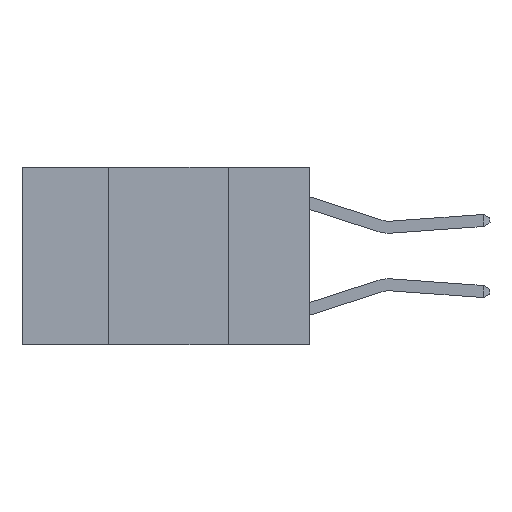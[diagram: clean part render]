
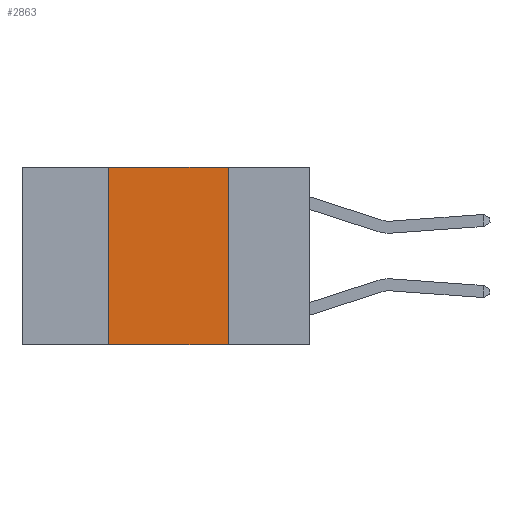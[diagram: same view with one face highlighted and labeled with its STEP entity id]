
A CAD part, left-side view. The second image highlights one B-rep face of the part: STEP entity #2863.
In plain terms, the highlighted planar face has unit normal (-1, 0, 0).
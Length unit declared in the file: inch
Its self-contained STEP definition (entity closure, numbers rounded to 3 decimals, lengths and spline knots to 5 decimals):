
#155 = VERTEX_POINT ( 'NONE', #14395 ) ;
#500 = DIRECTION ( 'NONE',  ( 0., -1., 0. ) ) ;
#673 = CARTESIAN_POINT ( 'NONE',  ( 0., 0.17, 0. ) ) ;
#902 = VERTEX_POINT ( 'NONE', #6313 ) ;
#1097 = VECTOR ( 'NONE', #13581, 39.37008 ) ;
#1198 = ORIENTED_EDGE ( 'NONE', *, *, #15885, .F. ) ;
#1408 = EDGE_CURVE ( 'NONE', #12619, #902, #13025, .T. ) ;
#2148 = DIRECTION ( 'NONE',  ( 0., 0., -1. ) ) ;
#2248 = EDGE_LOOP ( 'NONE', ( #1198, #7878, #8246, #12361 ) ) ;
#2275 = DIRECTION ( 'NONE',  ( 1., 0., 0. ) ) ;
#2738 = EDGE_CURVE ( 'NONE', #12619, #155, #17700, .T. ) ;
#2863 = ADVANCED_FACE ( 'NONE', ( #14900 ), #9788, .F. ) ;
#4066 = LINE ( 'NONE', #9412, #15125 ) ;
#4560 = CARTESIAN_POINT ( 'NONE',  ( 0., 0.6, 0. ) ) ;
#6313 = CARTESIAN_POINT ( 'NONE',  ( 0., 0.17, -0.37 ) ) ;
#7878 = ORIENTED_EDGE ( 'NONE', *, *, #15135, .F. ) ;
#8246 = ORIENTED_EDGE ( 'NONE', *, *, #2738, .F. ) ;
#9407 = VECTOR ( 'NONE', #2148, 39.37008 ) ;
#9412 = CARTESIAN_POINT ( 'NONE',  ( 0., 0.6, 0. ) ) ;
#9788 = PLANE ( 'NONE',  #14128 ) ;
#9894 = CARTESIAN_POINT ( 'NONE',  ( 0., 0.6, -0.37 ) ) ;
#9947 = CARTESIAN_POINT ( 'NONE',  ( 0., 0.42, 0. ) ) ;
#12361 = ORIENTED_EDGE ( 'NONE', *, *, #1408, .T. ) ;
#12619 = VERTEX_POINT ( 'NONE', #13382 ) ;
#13025 = LINE ( 'NONE', #9894, #1097 ) ;
#13382 = CARTESIAN_POINT ( 'NONE',  ( 0., 0.42, -0.37 ) ) ;
#13581 = DIRECTION ( 'NONE',  ( 0., -1., 0. ) ) ;
#14128 = AXIS2_PLACEMENT_3D ( 'NONE', #4560, #2275, #16400 ) ;
#14395 = CARTESIAN_POINT ( 'NONE',  ( 0., 0.42, 0. ) ) ;
#14596 = DIRECTION ( 'NONE',  ( 0., 0., 1. ) ) ;
#14900 = FACE_OUTER_BOUND ( 'NONE', #2248, .T. ) ;
#15125 = VECTOR ( 'NONE', #500, 39.37008 ) ;
#15135 = EDGE_CURVE ( 'NONE', #155, #18256, #4066, .T. ) ;
#15885 = EDGE_CURVE ( 'NONE', #18256, #902, #18352, .T. ) ;
#16400 = DIRECTION ( 'NONE',  ( 0., 0., -1. ) ) ;
#17700 = LINE ( 'NONE', #9947, #18164 ) ;
#18057 = CARTESIAN_POINT ( 'NONE',  ( 0., 0.17, 0. ) ) ;
#18164 = VECTOR ( 'NONE', #14596, 39.37008 ) ;
#18256 = VERTEX_POINT ( 'NONE', #18057 ) ;
#18352 = LINE ( 'NONE', #673, #9407 ) ;
